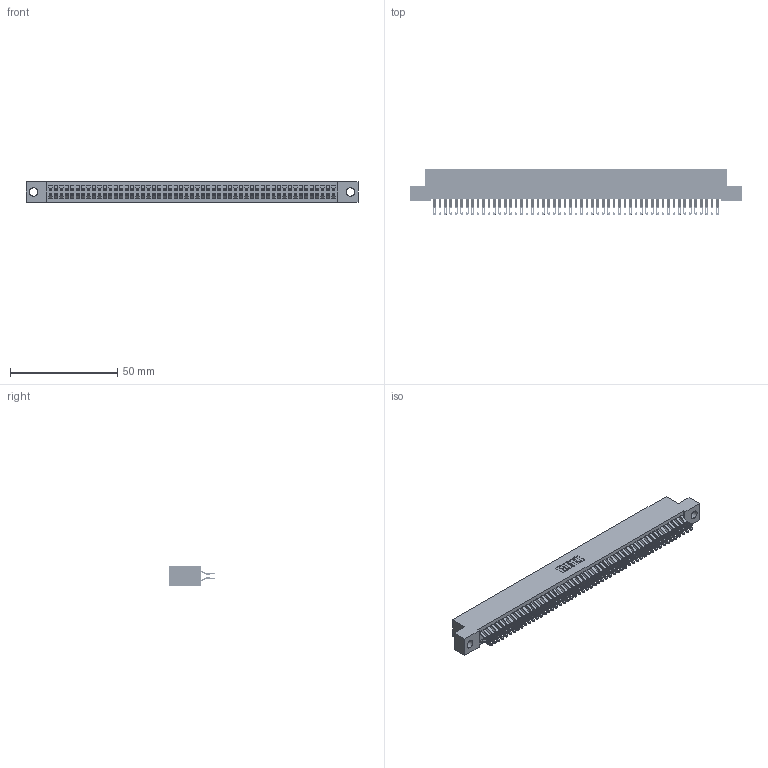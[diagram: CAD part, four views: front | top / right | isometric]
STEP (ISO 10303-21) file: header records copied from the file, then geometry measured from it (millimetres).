
FILE_DESCRIPTION (( 'STEP AP203' ), '1' );
FILE_NAME ('342-106-555-204.STEP', '2018-08-14T07:10:14', ( '' ), ( '' ), 'SwSTEP 2.0', 'SolidWorks 2016', '' );
FILE_SCHEMA (( 'CONFIG_CONTROL_DESIGN' ));
Length unit declared in the file: inch
Products named in the file (3): 342 Part_.156 TH; 345-292-001_555 Tail; 342-106-555-204
Assembly tree (107 placements, depth 2):
  342-106-555-204
    342 Part_.156 TH
    345-292-001_555 Tail  x106
Bounding box: 154.94 x 21.47 x 9.4 mm (x, y, z)
Volume: 14181 mm3; surface area: 24203.9 mm2
Topology: 107 solids, 107 shells, 6258 faces, 19697 edges, 13130 vertices
Faces by surface type: plane 3670, cylinder 2588
Entity records: 32871 total; most frequent: CARTESIAN_POINT 5468, ORIENTED_EDGE 5374, DIRECTION 4623, EDGE_CURVE 2687, VECTOR 2539, LINE 2539, VERTEX_POINT 1790, AXIS2_PLACEMENT_3D 1042
